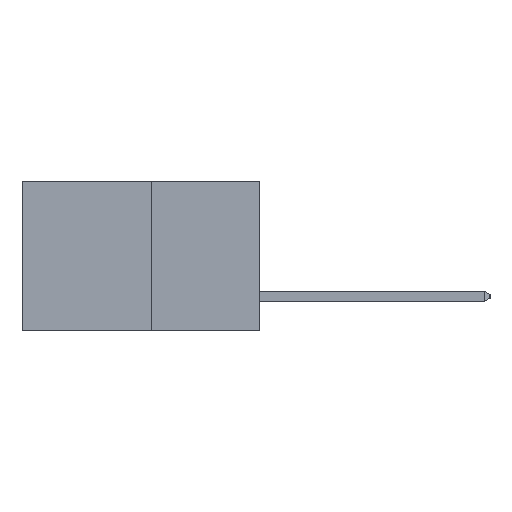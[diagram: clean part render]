
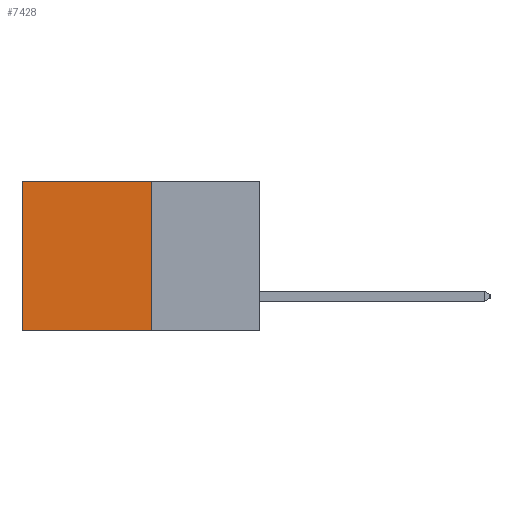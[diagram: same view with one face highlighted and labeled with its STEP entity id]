
A CAD part, left-side view. The second image highlights one B-rep face of the part: STEP entity #7428.
In plain terms, the highlighted planar face has unit normal (-1, 0, 0).
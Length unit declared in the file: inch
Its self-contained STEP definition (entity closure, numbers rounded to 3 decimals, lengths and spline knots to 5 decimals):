
#267 = CARTESIAN_POINT ( 'NONE',  ( 0.277, 0.59, 0. ) ) ;
#419 = VERTEX_POINT ( 'NONE', #267 ) ;
#621 = VECTOR ( 'NONE', #4089, 39.37008 ) ;
#1859 = EDGE_CURVE ( 'NONE', #5061, #2013, #12457, .T. ) ;
#2013 = VERTEX_POINT ( 'NONE', #9718 ) ;
#2601 = AXIS2_PLACEMENT_3D ( 'NONE', #6758, #6579, #6577 ) ;
#2634 = VECTOR ( 'NONE', #12712, 39.37008 ) ;
#3744 = VECTOR ( 'NONE', #7905, 39.37008 ) ;
#3995 = CARTESIAN_POINT ( 'NONE',  ( 0.277, 0.27, 0. ) ) ;
#4089 = DIRECTION ( 'NONE',  ( 0., 0., -1. ) ) ;
#4764 = EDGE_CURVE ( 'NONE', #5061, #419, #13881, .T. ) ;
#5061 = VERTEX_POINT ( 'NONE', #3995 ) ;
#6237 = DIRECTION ( 'NONE',  ( 0., 1., 0. ) ) ;
#6364 = EDGE_LOOP ( 'NONE', ( #10816, #15132, #15276, #11736 ) ) ;
#6577 = DIRECTION ( 'NONE',  ( 0., 0., -1. ) ) ;
#6579 = DIRECTION ( 'NONE',  ( 1., 0., 0. ) ) ;
#6691 = PLANE ( 'NONE',  #2601 ) ;
#6758 = CARTESIAN_POINT ( 'NONE',  ( 0.277, 0.27, -0.37 ) ) ;
#7428 = ADVANCED_FACE ( 'NONE', ( #12713 ), #6691, .F. ) ;
#7905 = DIRECTION ( 'NONE',  ( 0., 1., 0. ) ) ;
#8048 = CARTESIAN_POINT ( 'NONE',  ( 0.277, 0.27, 0. ) ) ;
#8419 = EDGE_CURVE ( 'NONE', #2013, #9642, #9188, .T. ) ;
#8516 = CARTESIAN_POINT ( 'NONE',  ( 0.277, 0.59, -0.37 ) ) ;
#9188 = LINE ( 'NONE', #13588, #12491 ) ;
#9642 = VERTEX_POINT ( 'NONE', #8516 ) ;
#9718 = CARTESIAN_POINT ( 'NONE',  ( 0.277, 0.27, -0.37 ) ) ;
#10160 = CARTESIAN_POINT ( 'NONE',  ( 0.277, 0.59, -0.37 ) ) ;
#10522 = LINE ( 'NONE', #10160, #621 ) ;
#10816 = ORIENTED_EDGE ( 'NONE', *, *, #11109, .T. ) ;
#11109 = EDGE_CURVE ( 'NONE', #419, #9642, #10522, .T. ) ;
#11736 = ORIENTED_EDGE ( 'NONE', *, *, #4764, .T. ) ;
#12457 = LINE ( 'NONE', #13031, #2634 ) ;
#12491 = VECTOR ( 'NONE', #6237, 39.37008 ) ;
#12712 = DIRECTION ( 'NONE',  ( 0., 0., -1. ) ) ;
#12713 = FACE_OUTER_BOUND ( 'NONE', #6364, .T. ) ;
#13031 = CARTESIAN_POINT ( 'NONE',  ( 0.277, 0.27, -0.37 ) ) ;
#13588 = CARTESIAN_POINT ( 'NONE',  ( 0.277, 0.27, -0.37 ) ) ;
#13881 = LINE ( 'NONE', #8048, #3744 ) ;
#15132 = ORIENTED_EDGE ( 'NONE', *, *, #8419, .F. ) ;
#15276 = ORIENTED_EDGE ( 'NONE', *, *, #1859, .F. ) ;
